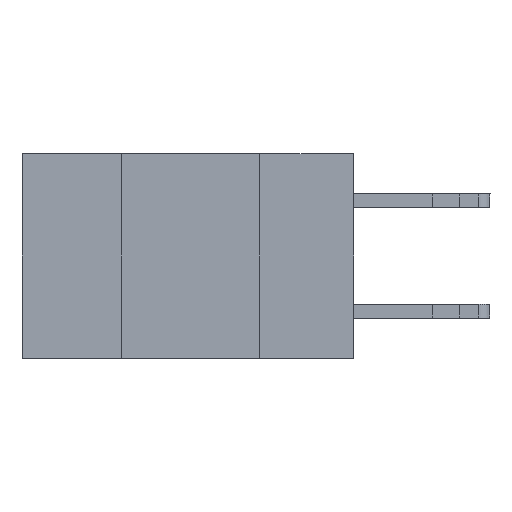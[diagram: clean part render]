
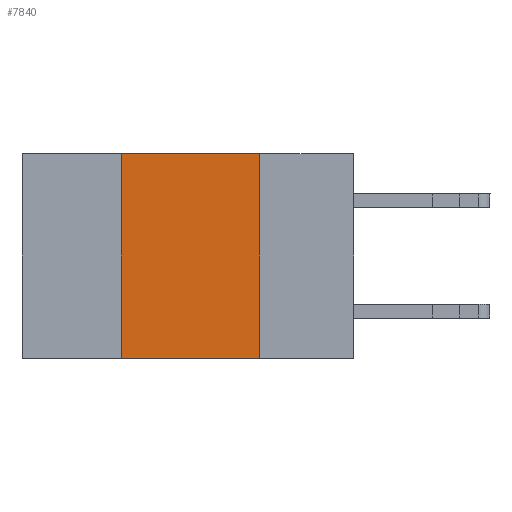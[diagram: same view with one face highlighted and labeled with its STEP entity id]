
A CAD part, left-side view. The second image highlights one B-rep face of the part: STEP entity #7840.
In plain terms, the highlighted planar face has unit normal (-1, 0, 0).
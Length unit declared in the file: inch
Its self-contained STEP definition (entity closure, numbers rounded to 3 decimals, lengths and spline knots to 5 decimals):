
#222 = ORIENTED_EDGE ( 'NONE', *, *, #15117, .F. ) ;
#1403 = EDGE_CURVE ( 'NONE', #14324, #2786, #10564, .T. ) ;
#2254 = FACE_OUTER_BOUND ( 'NONE', #20075, .T. ) ;
#2786 = VERTEX_POINT ( 'NONE', #5668 ) ;
#2974 = CARTESIAN_POINT ( 'NONE',  ( 0., 0.17, 0. ) ) ;
#3217 = EDGE_CURVE ( 'NONE', #17186, #14324, #18764, .T. ) ;
#3960 = DIRECTION ( 'NONE',  ( 0., -1., 0. ) ) ;
#4144 = DIRECTION ( 'NONE',  ( 0., 0., 1. ) ) ;
#5668 = CARTESIAN_POINT ( 'NONE',  ( 0., 0.17, 0. ) ) ;
#6633 = AXIS2_PLACEMENT_3D ( 'NONE', #18897, #15401, #18788 ) ;
#7572 = DIRECTION ( 'NONE',  ( 0., -1., 0. ) ) ;
#7840 = ADVANCED_FACE ( 'NONE', ( #2254 ), #10566, .F. ) ;
#9329 = ORIENTED_EDGE ( 'NONE', *, *, #17675, .T. ) ;
#10564 = LINE ( 'NONE', #20187, #19149 ) ;
#10566 = PLANE ( 'NONE',  #6633 ) ;
#11096 = CARTESIAN_POINT ( 'NONE',  ( 0., 0.17, -0.37 ) ) ;
#11959 = VECTOR ( 'NONE', #17002, 39.37008 ) ;
#12293 = LINE ( 'NONE', #2974, #11959 ) ;
#12698 = ORIENTED_EDGE ( 'NONE', *, *, #1403, .F. ) ;
#13765 = VECTOR ( 'NONE', #4144, 39.37008 ) ;
#14166 = CARTESIAN_POINT ( 'NONE',  ( 0., 0.42, 0. ) ) ;
#14324 = VERTEX_POINT ( 'NONE', #14166 ) ;
#15117 = EDGE_CURVE ( 'NONE', #2786, #20419, #12293, .T. ) ;
#15401 = DIRECTION ( 'NONE',  ( 1., 0., 0. ) ) ;
#15686 = CARTESIAN_POINT ( 'NONE',  ( 0., 0.42, 0. ) ) ;
#15928 = CARTESIAN_POINT ( 'NONE',  ( 0., 0.6, -0.37 ) ) ;
#17002 = DIRECTION ( 'NONE',  ( 0., 0., -1. ) ) ;
#17186 = VERTEX_POINT ( 'NONE', #19310 ) ;
#17401 = LINE ( 'NONE', #15928, #18497 ) ;
#17435 = ORIENTED_EDGE ( 'NONE', *, *, #3217, .F. ) ;
#17675 = EDGE_CURVE ( 'NONE', #17186, #20419, #17401, .T. ) ;
#18497 = VECTOR ( 'NONE', #7572, 39.37008 ) ;
#18764 = LINE ( 'NONE', #15686, #13765 ) ;
#18788 = DIRECTION ( 'NONE',  ( 0., 0., -1. ) ) ;
#18897 = CARTESIAN_POINT ( 'NONE',  ( 0., 0.6, 0. ) ) ;
#19149 = VECTOR ( 'NONE', #3960, 39.37008 ) ;
#19310 = CARTESIAN_POINT ( 'NONE',  ( 0., 0.42, -0.37 ) ) ;
#20075 = EDGE_LOOP ( 'NONE', ( #222, #12698, #17435, #9329 ) ) ;
#20187 = CARTESIAN_POINT ( 'NONE',  ( 0., 0.6, 0. ) ) ;
#20419 = VERTEX_POINT ( 'NONE', #11096 ) ;
